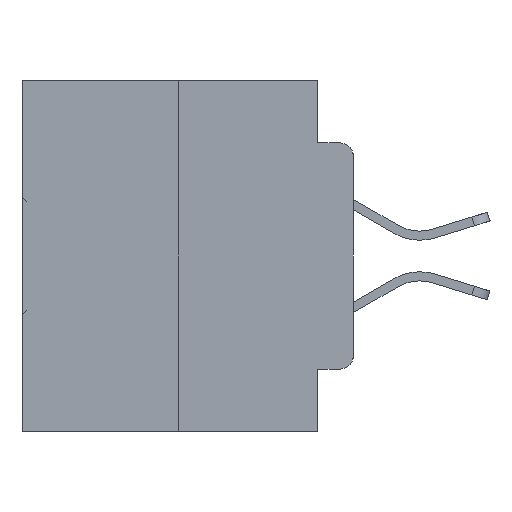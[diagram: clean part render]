
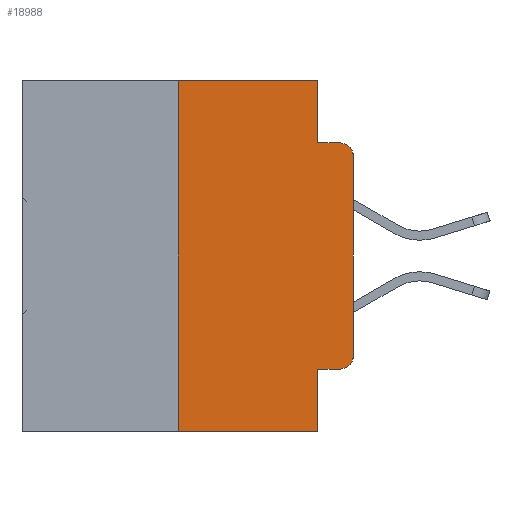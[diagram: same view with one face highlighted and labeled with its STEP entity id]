
A CAD part, left-side view. The second image highlights one B-rep face of the part: STEP entity #18988.
In plain terms, the highlighted planar face has unit normal (-1, 0, 0).
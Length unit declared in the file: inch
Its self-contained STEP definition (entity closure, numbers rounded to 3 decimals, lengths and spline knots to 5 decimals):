
#186 = EDGE_CURVE ( 'NONE', #30079, #26110, #12490, .T. ) ;
#1638 = ORIENTED_EDGE ( 'NONE', *, *, #11943, .F. ) ;
#1659 = FACE_OUTER_BOUND ( 'NONE', #21402, .T. ) ;
#2369 = CARTESIAN_POINT ( 'NONE',  ( 0., 0.051, -0.5 ) ) ;
#3180 = EDGE_CURVE ( 'NONE', #14676, #21595, #18948, .T. ) ;
#3465 = ORIENTED_EDGE ( 'NONE', *, *, #6832, .T. ) ;
#3625 = DIRECTION ( 'NONE',  ( 0., 0., -1. ) ) ;
#4113 = VERTEX_POINT ( 'NONE', #9508 ) ;
#4133 = EDGE_CURVE ( 'NONE', #8820, #14287, #31983, .T. ) ;
#4186 = AXIS2_PLACEMENT_3D ( 'NONE', #25171, #12354, #27329 ) ;
#4515 = DIRECTION ( 'NONE',  ( 0., 0., 1. ) ) ;
#4727 = ORIENTED_EDGE ( 'NONE', *, *, #3180, .F. ) ;
#4741 = LINE ( 'NONE', #5229, #18017 ) ;
#4766 = ORIENTED_EDGE ( 'NONE', *, *, #4133, .F. ) ;
#5045 = VECTOR ( 'NONE', #5499, 39.37008 ) ;
#5197 = VECTOR ( 'NONE', #32603, 39.37008 ) ;
#5229 = CARTESIAN_POINT ( 'NONE',  ( 0., 0.051, -0.0885 ) ) ;
#5499 = DIRECTION ( 'NONE',  ( 0., -1., 0. ) ) ;
#5520 = CARTESIAN_POINT ( 'NONE',  ( 0., 0.051, -0.0885 ) ) ;
#6363 = CARTESIAN_POINT ( 'NONE',  ( 0., 0.02, -0.4115 ) ) ;
#6686 = ORIENTED_EDGE ( 'NONE', *, *, #186, .T. ) ;
#6832 = EDGE_CURVE ( 'NONE', #17416, #30079, #17179, .T. ) ;
#7825 = CARTESIAN_POINT ( 'NONE',  ( 0., 0.051, -0.4115 ) ) ;
#8820 = VERTEX_POINT ( 'NONE', #18111 ) ;
#9150 = DIRECTION ( 'NONE',  ( 0., 0., -1. ) ) ;
#9508 = CARTESIAN_POINT ( 'NONE',  ( 0., 0.051, 0. ) ) ;
#9636 = CARTESIAN_POINT ( 'NONE',  ( 0., 0.473, 0. ) ) ;
#9861 = LINE ( 'NONE', #16876, #13063 ) ;
#10072 = DIRECTION ( 'NONE',  ( 0., 0., -1. ) ) ;
#11443 = ORIENTED_EDGE ( 'NONE', *, *, #22577, .T. ) ;
#11943 = EDGE_CURVE ( 'NONE', #29429, #26110, #4741, .T. ) ;
#12354 = DIRECTION ( 'NONE',  ( -1., 0., 0. ) ) ;
#12490 = CIRCLE ( 'NONE', #17839, 0.02 ) ;
#12551 = DIRECTION ( 'NONE',  ( 0., -1., 0. ) ) ;
#12611 = VECTOR ( 'NONE', #3625, 39.37008 ) ;
#13063 = VECTOR ( 'NONE', #29672, 39.37008 ) ;
#13298 = ORIENTED_EDGE ( 'NONE', *, *, #20716, .F. ) ;
#14148 = PLANE ( 'NONE',  #32093 ) ;
#14281 = CIRCLE ( 'NONE', #4186, 0.02 ) ;
#14287 = VERTEX_POINT ( 'NONE', #14550 ) ;
#14506 = VECTOR ( 'NONE', #4515, 39.37008 ) ;
#14550 = CARTESIAN_POINT ( 'NONE',  ( 0., 0.25, 0. ) ) ;
#14676 = VERTEX_POINT ( 'NONE', #17653 ) ;
#15469 = CARTESIAN_POINT ( 'NONE',  ( 0., 0.02, -0.0885 ) ) ;
#16498 = CARTESIAN_POINT ( 'NONE',  ( 0., 0.473, -0.5 ) ) ;
#16582 = VECTOR ( 'NONE', #21482, 39.37008 ) ;
#16876 = CARTESIAN_POINT ( 'NONE',  ( 0., 0.473, 0. ) ) ;
#16958 = CARTESIAN_POINT ( 'NONE',  ( 0., 0., -0.1085 ) ) ;
#17179 = LINE ( 'NONE', #22508, #14506 ) ;
#17416 = VERTEX_POINT ( 'NONE', #23599 ) ;
#17653 = CARTESIAN_POINT ( 'NONE',  ( 0., 0.051, -0.4115 ) ) ;
#17839 = AXIS2_PLACEMENT_3D ( 'NONE', #32862, #29873, #10072 ) ;
#18017 = VECTOR ( 'NONE', #12551, 39.37008 ) ;
#18111 = CARTESIAN_POINT ( 'NONE',  ( 0., 0.25, -0.5 ) ) ;
#18948 = LINE ( 'NONE', #21453, #12611 ) ;
#18988 = ADVANCED_FACE ( 'NONE', ( #1659 ), #14148, .F. ) ;
#19305 = ORIENTED_EDGE ( 'NONE', *, *, #19928, .T. ) ;
#19928 = EDGE_CURVE ( 'NONE', #14676, #29141, #20175, .T. ) ;
#20175 = LINE ( 'NONE', #7825, #5045 ) ;
#20716 = EDGE_CURVE ( 'NONE', #14287, #4113, #9861, .T. ) ;
#20994 = LINE ( 'NONE', #31131, #16582 ) ;
#20996 = VECTOR ( 'NONE', #24495, 39.37008 ) ;
#21402 = EDGE_LOOP ( 'NONE', ( #3465, #6686, #1638, #31360, #13298, #4766, #11443, #4727, #19305, #21878 ) ) ;
#21453 = CARTESIAN_POINT ( 'NONE',  ( 0., 0.051, 0. ) ) ;
#21482 = DIRECTION ( 'NONE',  ( 0., 0., -1. ) ) ;
#21595 = VERTEX_POINT ( 'NONE', #2369 ) ;
#21878 = ORIENTED_EDGE ( 'NONE', *, *, #27965, .T. ) ;
#22508 = CARTESIAN_POINT ( 'NONE',  ( 0., 0., 0. ) ) ;
#22577 = EDGE_CURVE ( 'NONE', #8820, #21595, #29122, .T. ) ;
#23599 = CARTESIAN_POINT ( 'NONE',  ( 0., 0., -0.3915 ) ) ;
#24495 = DIRECTION ( 'NONE',  ( 0., 0., 1. ) ) ;
#25165 = CARTESIAN_POINT ( 'NONE',  ( 0., 0.25, 0. ) ) ;
#25171 = CARTESIAN_POINT ( 'NONE',  ( 0., 0.02, -0.3915 ) ) ;
#26110 = VERTEX_POINT ( 'NONE', #15469 ) ;
#27329 = DIRECTION ( 'NONE',  ( 0., 0., -1. ) ) ;
#27965 = EDGE_CURVE ( 'NONE', #29141, #17416, #14281, .T. ) ;
#29122 = LINE ( 'NONE', #16498, #5197 ) ;
#29141 = VERTEX_POINT ( 'NONE', #6363 ) ;
#29429 = VERTEX_POINT ( 'NONE', #5520 ) ;
#29672 = DIRECTION ( 'NONE',  ( 0., -1., 0. ) ) ;
#29873 = DIRECTION ( 'NONE',  ( -1., 0., 0. ) ) ;
#30079 = VERTEX_POINT ( 'NONE', #16958 ) ;
#31131 = CARTESIAN_POINT ( 'NONE',  ( 0., 0.051, 0. ) ) ;
#31360 = ORIENTED_EDGE ( 'NONE', *, *, #32501, .F. ) ;
#31941 = DIRECTION ( 'NONE',  ( 1., 0., 0. ) ) ;
#31983 = LINE ( 'NONE', #25165, #20996 ) ;
#32093 = AXIS2_PLACEMENT_3D ( 'NONE', #9636, #31941, #9150 ) ;
#32501 = EDGE_CURVE ( 'NONE', #4113, #29429, #20994, .T. ) ;
#32603 = DIRECTION ( 'NONE',  ( 0., -1., 0. ) ) ;
#32862 = CARTESIAN_POINT ( 'NONE',  ( 0., 0.02, -0.1085 ) ) ;
